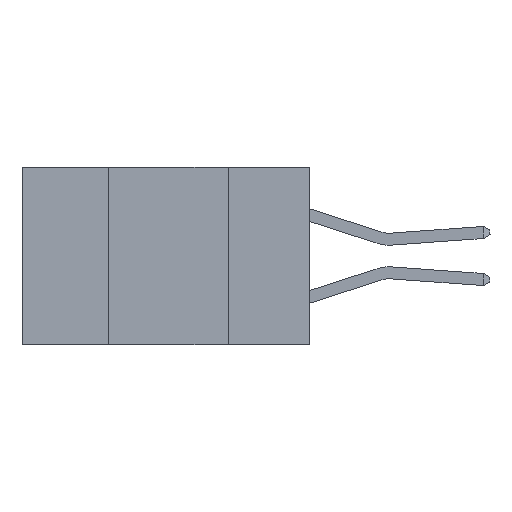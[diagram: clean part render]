
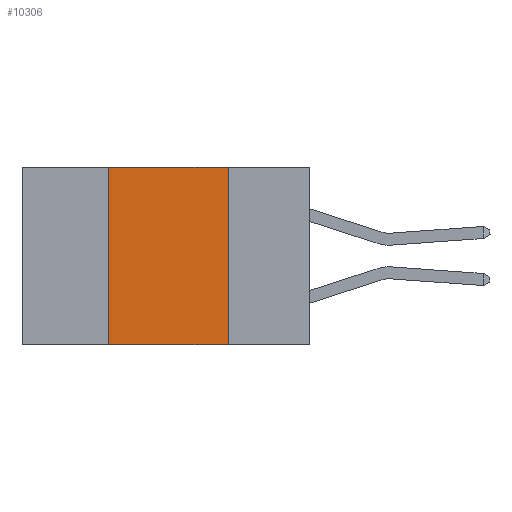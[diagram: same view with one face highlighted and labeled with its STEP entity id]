
A CAD part, left-side view. The second image highlights one B-rep face of the part: STEP entity #10306.
In plain terms, the highlighted planar face has unit normal (-1, 0, 0).
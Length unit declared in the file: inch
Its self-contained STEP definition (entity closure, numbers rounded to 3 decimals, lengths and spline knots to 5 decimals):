
#685 = DIRECTION ( 'NONE',  ( 0., 0., -1. ) ) ;
#873 = DIRECTION ( 'NONE',  ( 0., -1., 0. ) ) ;
#1829 = CARTESIAN_POINT ( 'NONE',  ( 0., 0.42, -0.37 ) ) ;
#2024 = VECTOR ( 'NONE', #20344, 39.37008 ) ;
#2264 = CARTESIAN_POINT ( 'NONE',  ( 0., 0.42, 0. ) ) ;
#2577 = CARTESIAN_POINT ( 'NONE',  ( 0., 0.42, -0.37 ) ) ;
#2882 = LINE ( 'NONE', #2577, #8799 ) ;
#3467 = AXIS2_PLACEMENT_3D ( 'NONE', #16846, #3908, #685 ) ;
#3908 = DIRECTION ( 'NONE',  ( 1., 0., 0. ) ) ;
#4080 = EDGE_CURVE ( 'NONE', #13648, #17890, #4098, .T. ) ;
#4098 = LINE ( 'NONE', #16826, #4666 ) ;
#4335 = CARTESIAN_POINT ( 'NONE',  ( 0., 0.17, -0.37 ) ) ;
#4602 = EDGE_CURVE ( 'NONE', #19040, #18669, #7698, .T. ) ;
#4666 = VECTOR ( 'NONE', #873, 39.37008 ) ;
#5301 = LINE ( 'NONE', #14912, #12563 ) ;
#7395 = ORIENTED_EDGE ( 'NONE', *, *, #4602, .F. ) ;
#7553 = ORIENTED_EDGE ( 'NONE', *, *, #11600, .F. ) ;
#7698 = LINE ( 'NONE', #15759, #2024 ) ;
#8584 = FACE_OUTER_BOUND ( 'NONE', #9190, .T. ) ;
#8799 = VECTOR ( 'NONE', #10803, 39.37008 ) ;
#9190 = EDGE_LOOP ( 'NONE', ( #13193, #7395, #7553, #17855 ) ) ;
#10306 = ADVANCED_FACE ( 'NONE', ( #8584 ), #14960, .F. ) ;
#10803 = DIRECTION ( 'NONE',  ( 0., 0., 1. ) ) ;
#11600 = EDGE_CURVE ( 'NONE', #13648, #19040, #2882, .T. ) ;
#12563 = VECTOR ( 'NONE', #13239, 39.37008 ) ;
#13193 = ORIENTED_EDGE ( 'NONE', *, *, #14267, .F. ) ;
#13239 = DIRECTION ( 'NONE',  ( 0., 0., -1. ) ) ;
#13648 = VERTEX_POINT ( 'NONE', #1829 ) ;
#14267 = EDGE_CURVE ( 'NONE', #18669, #17890, #5301, .T. ) ;
#14427 = CARTESIAN_POINT ( 'NONE',  ( 0., 0.17, 0. ) ) ;
#14912 = CARTESIAN_POINT ( 'NONE',  ( 0., 0.17, -0.37 ) ) ;
#14960 = PLANE ( 'NONE',  #3467 ) ;
#15759 = CARTESIAN_POINT ( 'NONE',  ( 0., 0.6, 0. ) ) ;
#16826 = CARTESIAN_POINT ( 'NONE',  ( 0., 0.6, -0.37 ) ) ;
#16846 = CARTESIAN_POINT ( 'NONE',  ( 0., 0.6, 0. ) ) ;
#17855 = ORIENTED_EDGE ( 'NONE', *, *, #4080, .T. ) ;
#17890 = VERTEX_POINT ( 'NONE', #4335 ) ;
#18669 = VERTEX_POINT ( 'NONE', #14427 ) ;
#19040 = VERTEX_POINT ( 'NONE', #2264 ) ;
#20344 = DIRECTION ( 'NONE',  ( 0., -1., 0. ) ) ;
